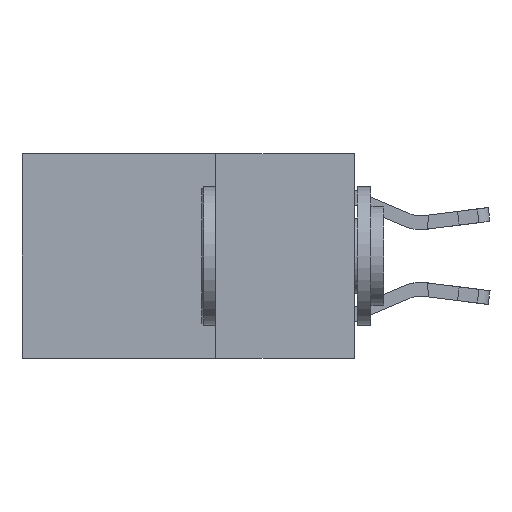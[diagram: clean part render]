
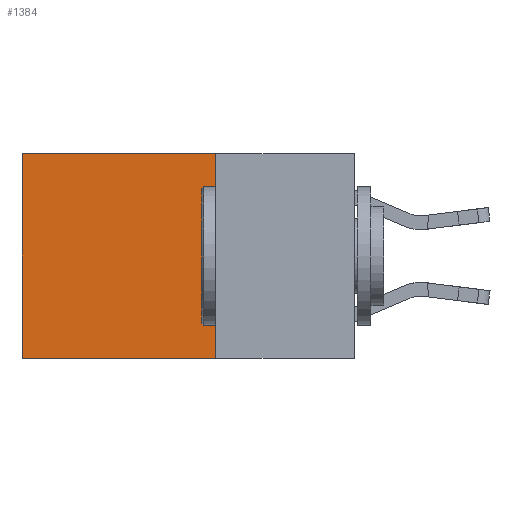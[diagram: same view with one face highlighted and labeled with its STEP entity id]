
A CAD part, left-side view. The second image highlights one B-rep face of the part: STEP entity #1384.
In plain terms, the highlighted planar face has unit normal (-1, 0, 0).
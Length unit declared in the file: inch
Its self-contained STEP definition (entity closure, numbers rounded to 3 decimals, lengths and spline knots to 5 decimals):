
#671 = EDGE_CURVE ( 'NONE', #7831, #13078, #13260, .T. ) ;
#867 = PLANE ( 'NONE',  #15431 ) ;
#1010 = EDGE_LOOP ( 'NONE', ( #10067, #3537, #7297, #10986 ) ) ;
#1384 = ADVANCED_FACE ( 'NONE', ( #6167 ), #867, .F. ) ;
#2040 = VECTOR ( 'NONE', #13110, 39.37008 ) ;
#2292 = DIRECTION ( 'NONE',  ( 0., 0., -1. ) ) ;
#3410 = CARTESIAN_POINT ( 'NONE',  ( 0.2625, 0.6, -0.37 ) ) ;
#3537 = ORIENTED_EDGE ( 'NONE', *, *, #3728, .F. ) ;
#3728 = EDGE_CURVE ( 'NONE', #14782, #13078, #9654, .T. ) ;
#4451 = LINE ( 'NONE', #6238, #10722 ) ;
#4869 = CARTESIAN_POINT ( 'NONE',  ( 0.2625, 0.6, 0. ) ) ;
#6167 = FACE_OUTER_BOUND ( 'NONE', #1010, .T. ) ;
#6207 = VERTEX_POINT ( 'NONE', #14880 ) ;
#6238 = CARTESIAN_POINT ( 'NONE',  ( 0.2625, 0.25, 0. ) ) ;
#6306 = VECTOR ( 'NONE', #6925, 39.37008 ) ;
#6925 = DIRECTION ( 'NONE',  ( 0., 1., 0. ) ) ;
#7297 = ORIENTED_EDGE ( 'NONE', *, *, #13637, .F. ) ;
#7515 = DIRECTION ( 'NONE',  ( 0., 1., 0. ) ) ;
#7831 = VERTEX_POINT ( 'NONE', #4869 ) ;
#8223 = CARTESIAN_POINT ( 'NONE',  ( 0.2625, 0.25, 0. ) ) ;
#8632 = CARTESIAN_POINT ( 'NONE',  ( 0.2625, 0.25, 0. ) ) ;
#9542 = CARTESIAN_POINT ( 'NONE',  ( 0.2625, 0.6, 0. ) ) ;
#9545 = DIRECTION ( 'NONE',  ( 0., 0., -1. ) ) ;
#9654 = LINE ( 'NONE', #15564, #6306 ) ;
#9876 = DIRECTION ( 'NONE',  ( 1., 0., 0. ) ) ;
#10067 = ORIENTED_EDGE ( 'NONE', *, *, #671, .T. ) ;
#10722 = VECTOR ( 'NONE', #7515, 39.37008 ) ;
#10986 = ORIENTED_EDGE ( 'NONE', *, *, #13975, .T. ) ;
#13078 = VERTEX_POINT ( 'NONE', #3410 ) ;
#13110 = DIRECTION ( 'NONE',  ( 0., 0., -1. ) ) ;
#13260 = LINE ( 'NONE', #9542, #15372 ) ;
#13594 = CARTESIAN_POINT ( 'NONE',  ( 0.2625, 0.25, -0.37 ) ) ;
#13637 = EDGE_CURVE ( 'NONE', #6207, #14782, #14948, .T. ) ;
#13975 = EDGE_CURVE ( 'NONE', #6207, #7831, #4451, .T. ) ;
#14782 = VERTEX_POINT ( 'NONE', #13594 ) ;
#14880 = CARTESIAN_POINT ( 'NONE',  ( 0.2625, 0.25, 0. ) ) ;
#14948 = LINE ( 'NONE', #8223, #2040 ) ;
#15372 = VECTOR ( 'NONE', #9545, 39.37008 ) ;
#15431 = AXIS2_PLACEMENT_3D ( 'NONE', #8632, #9876, #2292 ) ;
#15564 = CARTESIAN_POINT ( 'NONE',  ( 0.2625, 0.25, -0.37 ) ) ;
